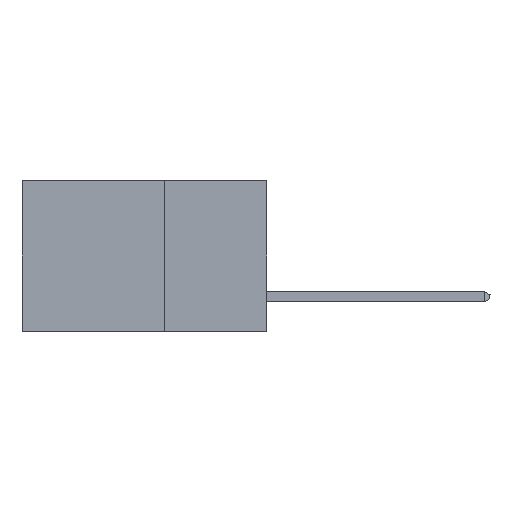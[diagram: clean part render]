
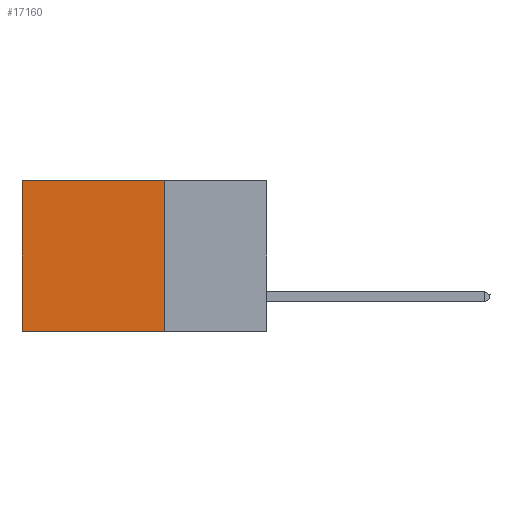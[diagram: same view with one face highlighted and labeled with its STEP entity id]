
A CAD part, left-side view. The second image highlights one B-rep face of the part: STEP entity #17160.
In plain terms, the highlighted planar face has unit normal (-1, 0, 0).
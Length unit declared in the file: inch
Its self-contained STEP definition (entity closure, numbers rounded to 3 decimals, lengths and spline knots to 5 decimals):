
#324 = EDGE_CURVE ( 'NONE', #16969, #5958, #1311, .T. ) ;
#657 = LINE ( 'NONE', #7251, #14555 ) ;
#1311 = LINE ( 'NONE', #6300, #17932 ) ;
#3069 = ORIENTED_EDGE ( 'NONE', *, *, #13919, .F. ) ;
#4111 = EDGE_CURVE ( 'NONE', #16969, #5760, #21236, .T. ) ;
#4114 = ORIENTED_EDGE ( 'NONE', *, *, #15024, .T. ) ;
#4675 = DIRECTION ( 'NONE',  ( 0., 1., 0. ) ) ;
#4962 = CARTESIAN_POINT ( 'NONE',  ( 0.2875, 0.6, 0. ) ) ;
#5459 = DIRECTION ( 'NONE',  ( 0., 0., -1. ) ) ;
#5760 = VERTEX_POINT ( 'NONE', #8316 ) ;
#5958 = VERTEX_POINT ( 'NONE', #6233 ) ;
#6233 = CARTESIAN_POINT ( 'NONE',  ( 0.2875, 0.6, 0. ) ) ;
#6300 = CARTESIAN_POINT ( 'NONE',  ( 0.2875, 0.25, 0. ) ) ;
#6806 = CARTESIAN_POINT ( 'NONE',  ( 0.2875, 0.25, 0. ) ) ;
#7251 = CARTESIAN_POINT ( 'NONE',  ( 0.2875, 0.25, -0.37 ) ) ;
#8316 = CARTESIAN_POINT ( 'NONE',  ( 0.2875, 0.25, -0.37 ) ) ;
#10536 = EDGE_LOOP ( 'NONE', ( #4114, #3069, #15814, #14917 ) ) ;
#12110 = FACE_OUTER_BOUND ( 'NONE', #10536, .T. ) ;
#13270 = CARTESIAN_POINT ( 'NONE',  ( 0.2875, 0.25, 0. ) ) ;
#13833 = DIRECTION ( 'NONE',  ( 1., 0., 0. ) ) ;
#13919 = EDGE_CURVE ( 'NONE', #5760, #18757, #657, .T. ) ;
#13927 = AXIS2_PLACEMENT_3D ( 'NONE', #6806, #13833, #20870 ) ;
#14325 = CARTESIAN_POINT ( 'NONE',  ( 0.2875, 0.25, 0. ) ) ;
#14555 = VECTOR ( 'NONE', #19801, 39.37008 ) ;
#14744 = CARTESIAN_POINT ( 'NONE',  ( 0.2875, 0.6, -0.37 ) ) ;
#14917 = ORIENTED_EDGE ( 'NONE', *, *, #324, .T. ) ;
#15024 = EDGE_CURVE ( 'NONE', #5958, #18757, #18895, .T. ) ;
#15324 = DIRECTION ( 'NONE',  ( 0., 0., -1. ) ) ;
#15559 = PLANE ( 'NONE',  #13927 ) ;
#15814 = ORIENTED_EDGE ( 'NONE', *, *, #4111, .F. ) ;
#16429 = VECTOR ( 'NONE', #15324, 39.37008 ) ;
#16969 = VERTEX_POINT ( 'NONE', #13270 ) ;
#17160 = ADVANCED_FACE ( 'NONE', ( #12110 ), #15559, .F. ) ;
#17932 = VECTOR ( 'NONE', #4675, 39.37008 ) ;
#18757 = VERTEX_POINT ( 'NONE', #14744 ) ;
#18895 = LINE ( 'NONE', #4962, #16429 ) ;
#19801 = DIRECTION ( 'NONE',  ( 0., 1., 0. ) ) ;
#20870 = DIRECTION ( 'NONE',  ( 0., 0., -1. ) ) ;
#21236 = LINE ( 'NONE', #14325, #21530 ) ;
#21530 = VECTOR ( 'NONE', #5459, 39.37008 ) ;
